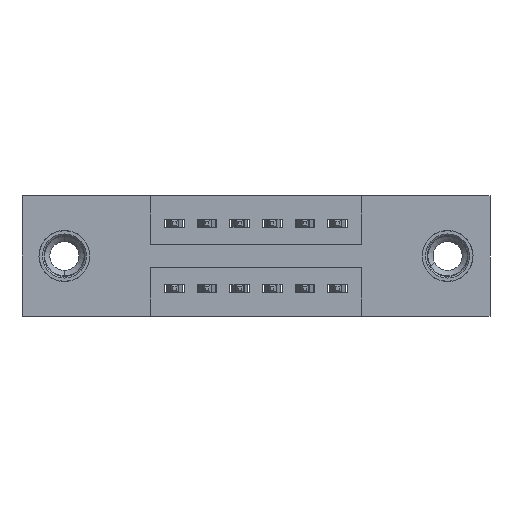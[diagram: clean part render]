
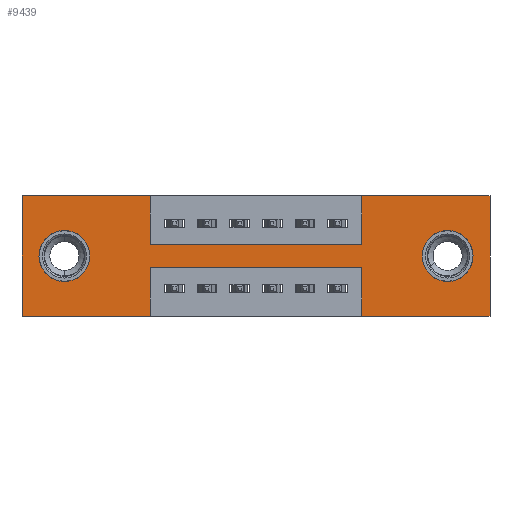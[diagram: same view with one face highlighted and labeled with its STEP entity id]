
A CAD part, front view. The second image highlights one B-rep face of the part: STEP entity #9439.
In plain terms, the highlighted planar face has unit normal (0, -1, 0).
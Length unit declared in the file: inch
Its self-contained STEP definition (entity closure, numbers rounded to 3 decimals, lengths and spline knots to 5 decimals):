
#86 = VERTEX_POINT ( 'NONE', #9624 ) ;
#166 = CARTESIAN_POINT ( 'NONE',  ( 1.305, 0., -0.107 ) ) ;
#255 = LINE ( 'NONE', #271, #2035 ) ;
#271 = CARTESIAN_POINT ( 'NONE',  ( 0., 0., -0.37 ) ) ;
#305 = DIRECTION ( 'NONE',  ( 0., 1., 0. ) ) ;
#328 = EDGE_CURVE ( 'NONE', #8763, #6198, #1957, .T. ) ;
#438 = CARTESIAN_POINT ( 'NONE',  ( 0., 0., -0.37 ) ) ;
#487 = EDGE_CURVE ( 'NONE', #9797, #8559, #4490, .T. ) ;
#551 = DIRECTION ( 'NONE',  ( 0., 0., 1. ) ) ;
#557 = EDGE_CURVE ( 'NONE', #3294, #9797, #3960, .T. ) ;
#584 = LINE ( 'NONE', #10082, #9208 ) ;
#622 = VERTEX_POINT ( 'NONE', #3909 ) ;
#624 = DIRECTION ( 'NONE',  ( 0., 0., -1. ) ) ;
#631 = CARTESIAN_POINT ( 'NONE',  ( 1.435, 0., 0. ) ) ;
#964 = AXIS2_PLACEMENT_3D ( 'NONE', #2836, #305, #3231 ) ;
#1215 = DIRECTION ( 'NONE',  ( 0., 1., 0. ) ) ;
#1253 = CARTESIAN_POINT ( 'NONE',  ( 1.0425, 0., -0.37 ) ) ;
#1307 = CARTESIAN_POINT ( 'NONE',  ( 0., 0., 0. ) ) ;
#1311 = VERTEX_POINT ( 'NONE', #1877 ) ;
#1319 = EDGE_LOOP ( 'NONE', ( #7394, #8394 ) ) ;
#1360 = VECTOR ( 'NONE', #5680, 39.37008 ) ;
#1423 = EDGE_CURVE ( 'NONE', #2237, #2375, #4762, .T. ) ;
#1459 = CARTESIAN_POINT ( 'NONE',  ( 0., 0., -0.37 ) ) ;
#1577 = LINE ( 'NONE', #1459, #7992 ) ;
#1595 = CIRCLE ( 'NONE', #5994, 0.078 ) ;
#1633 = EDGE_CURVE ( 'NONE', #3904, #86, #584, .T. ) ;
#1877 = CARTESIAN_POINT ( 'NONE',  ( 1.435, 0., -0.37 ) ) ;
#1957 = CIRCLE ( 'NONE', #10383, 0.078 ) ;
#1965 = VECTOR ( 'NONE', #6711, 39.37008 ) ;
#2035 = VECTOR ( 'NONE', #6252, 39.37008 ) ;
#2062 = LINE ( 'NONE', #9453, #10078 ) ;
#2091 = CARTESIAN_POINT ( 'NONE',  ( 0., 0., 0. ) ) ;
#2122 = VERTEX_POINT ( 'NONE', #5697 ) ;
#2140 = ORIENTED_EDGE ( 'NONE', *, *, #9640, .F. ) ;
#2146 = VERTEX_POINT ( 'NONE', #166 ) ;
#2157 = LINE ( 'NONE', #2091, #8541 ) ;
#2207 = EDGE_CURVE ( 'NONE', #86, #2122, #2062, .T. ) ;
#2211 = FACE_BOUND ( 'NONE', #1319, .T. ) ;
#2237 = VERTEX_POINT ( 'NONE', #9312 ) ;
#2335 = CARTESIAN_POINT ( 'NONE',  ( 0.3925, 0., 0. ) ) ;
#2375 = VERTEX_POINT ( 'NONE', #4013 ) ;
#2468 = VECTOR ( 'NONE', #4697, 39.37008 ) ;
#2488 = VERTEX_POINT ( 'NONE', #10717 ) ;
#2558 = DIRECTION ( 'NONE',  ( 0., 1., 0. ) ) ;
#2757 = CARTESIAN_POINT ( 'NONE',  ( 0.13, 0., -0.185 ) ) ;
#2765 = EDGE_CURVE ( 'NONE', #2146, #7243, #5010, .T. ) ;
#2836 = CARTESIAN_POINT ( 'NONE',  ( 1.305, 0., -0.185 ) ) ;
#2976 = DIRECTION ( 'NONE',  ( 0., 0., 1. ) ) ;
#3026 = CARTESIAN_POINT ( 'NONE',  ( 1.305, 0., -0.263 ) ) ;
#3231 = DIRECTION ( 'NONE',  ( 0., 0., -1. ) ) ;
#3263 = CARTESIAN_POINT ( 'NONE',  ( 0.13, 0., -0.107 ) ) ;
#3294 = VERTEX_POINT ( 'NONE', #8430 ) ;
#3357 = VECTOR ( 'NONE', #5086, 39.37008 ) ;
#3497 = LINE ( 'NONE', #1253, #9552 ) ;
#3625 = DIRECTION ( 'NONE',  ( 0., 0., 1. ) ) ;
#3855 = EDGE_CURVE ( 'NONE', #8559, #1311, #10166, .T. ) ;
#3904 = VERTEX_POINT ( 'NONE', #5490 ) ;
#3909 = CARTESIAN_POINT ( 'NONE',  ( 0., 0., 0. ) ) ;
#3960 = LINE ( 'NONE', #7753, #1965 ) ;
#4013 = CARTESIAN_POINT ( 'NONE',  ( 0.3925, 0., -0.15 ) ) ;
#4252 = ORIENTED_EDGE ( 'NONE', *, *, #4639, .F. ) ;
#4260 = EDGE_CURVE ( 'NONE', #2375, #3294, #8279, .T. ) ;
#4428 = DIRECTION ( 'NONE',  ( 0., -1., 0. ) ) ;
#4490 = LINE ( 'NONE', #7725, #8617 ) ;
#4499 = EDGE_LOOP ( 'NONE', ( #5506, #5507 ) ) ;
#4639 = EDGE_CURVE ( 'NONE', #2122, #8376, #255, .T. ) ;
#4697 = DIRECTION ( 'NONE',  ( 0., 0., -1. ) ) ;
#4762 = LINE ( 'NONE', #2335, #2468 ) ;
#5010 = CIRCLE ( 'NONE', #964, 0.078 ) ;
#5086 = DIRECTION ( 'NONE',  ( 0., 0., -1. ) ) ;
#5281 = CARTESIAN_POINT ( 'NONE',  ( 0., 0., -0.37 ) ) ;
#5383 = ORIENTED_EDGE ( 'NONE', *, *, #5393, .F. ) ;
#5393 = EDGE_CURVE ( 'NONE', #622, #2237, #2157, .T. ) ;
#5490 = CARTESIAN_POINT ( 'NONE',  ( 1.0425, 0., -0.22 ) ) ;
#5506 = ORIENTED_EDGE ( 'NONE', *, *, #2765, .T. ) ;
#5507 = ORIENTED_EDGE ( 'NONE', *, *, #8921, .T. ) ;
#5510 = DIRECTION ( 'NONE',  ( 1., 0., 0. ) ) ;
#5520 = ORIENTED_EDGE ( 'NONE', *, *, #2207, .F. ) ;
#5680 = DIRECTION ( 'NONE',  ( 1., 0., 0. ) ) ;
#5697 = CARTESIAN_POINT ( 'NONE',  ( 0.3925, 0., -0.37 ) ) ;
#5874 = EDGE_LOOP ( 'NONE', ( #5520, #6567, #6012, #9488, #7519, #8018, #7683, #7933, #6992, #5383, #2140, #4252 ) ) ;
#5994 = AXIS2_PLACEMENT_3D ( 'NONE', #2757, #8583, #3625 ) ;
#6012 = ORIENTED_EDGE ( 'NONE', *, *, #10746, .F. ) ;
#6198 = VERTEX_POINT ( 'NONE', #3263 ) ;
#6252 = DIRECTION ( 'NONE',  ( -1., 0., 0. ) ) ;
#6277 = CARTESIAN_POINT ( 'NONE',  ( 1.305, 0., -0.185 ) ) ;
#6309 = DIRECTION ( 'NONE',  ( 0., 0., 1. ) ) ;
#6567 = ORIENTED_EDGE ( 'NONE', *, *, #1633, .F. ) ;
#6635 = CARTESIAN_POINT ( 'NONE',  ( 1.435, 0., 0. ) ) ;
#6711 = DIRECTION ( 'NONE',  ( 0., 0., 1. ) ) ;
#6794 = LINE ( 'NONE', #1307, #10561 ) ;
#6926 = CARTESIAN_POINT ( 'NONE',  ( 0.13, 0., -0.185 ) ) ;
#6992 = ORIENTED_EDGE ( 'NONE', *, *, #1423, .F. ) ;
#6998 = EDGE_CURVE ( 'NONE', #6198, #8763, #1595, .T. ) ;
#7068 = DIRECTION ( 'NONE',  ( 0., 0., -1. ) ) ;
#7243 = VERTEX_POINT ( 'NONE', #3026 ) ;
#7394 = ORIENTED_EDGE ( 'NONE', *, *, #6998, .T. ) ;
#7519 = ORIENTED_EDGE ( 'NONE', *, *, #3855, .F. ) ;
#7683 = ORIENTED_EDGE ( 'NONE', *, *, #557, .F. ) ;
#7697 = AXIS2_PLACEMENT_3D ( 'NONE', #5281, #4428, #10136 ) ;
#7725 = CARTESIAN_POINT ( 'NONE',  ( 0., 0., 0. ) ) ;
#7753 = CARTESIAN_POINT ( 'NONE',  ( 1.0425, 0., 0. ) ) ;
#7933 = ORIENTED_EDGE ( 'NONE', *, *, #4260, .F. ) ;
#7956 = EDGE_CURVE ( 'NONE', #1311, #2488, #1577, .T. ) ;
#7992 = VECTOR ( 'NONE', #8952, 39.37008 ) ;
#8018 = ORIENTED_EDGE ( 'NONE', *, *, #487, .F. ) ;
#8137 = DIRECTION ( 'NONE',  ( -1., 0., 0. ) ) ;
#8279 = LINE ( 'NONE', #10456, #1360 ) ;
#8376 = VERTEX_POINT ( 'NONE', #438 ) ;
#8394 = ORIENTED_EDGE ( 'NONE', *, *, #328, .T. ) ;
#8430 = CARTESIAN_POINT ( 'NONE',  ( 1.0425, 0., -0.15 ) ) ;
#8541 = VECTOR ( 'NONE', #5510, 39.37008 ) ;
#8559 = VERTEX_POINT ( 'NONE', #631 ) ;
#8583 = DIRECTION ( 'NONE',  ( 0., 1., 0. ) ) ;
#8589 = FACE_BOUND ( 'NONE', #4499, .T. ) ;
#8617 = VECTOR ( 'NONE', #9157, 39.37008 ) ;
#8763 = VERTEX_POINT ( 'NONE', #9207 ) ;
#8849 = FACE_OUTER_BOUND ( 'NONE', #5874, .T. ) ;
#8921 = EDGE_CURVE ( 'NONE', #7243, #2146, #9591, .T. ) ;
#8952 = DIRECTION ( 'NONE',  ( -1., 0., 0. ) ) ;
#8987 = CARTESIAN_POINT ( 'NONE',  ( 1.0425, 0., 0. ) ) ;
#9157 = DIRECTION ( 'NONE',  ( 1., 0., 0. ) ) ;
#9207 = CARTESIAN_POINT ( 'NONE',  ( 0.13, 0., -0.263 ) ) ;
#9208 = VECTOR ( 'NONE', #8137, 39.37008 ) ;
#9312 = CARTESIAN_POINT ( 'NONE',  ( 0.3925, 0., 0. ) ) ;
#9333 = PLANE ( 'NONE',  #7697 ) ;
#9439 = ADVANCED_FACE ( 'NONE', ( #8589, #2211, #8849 ), #9333, .T. ) ;
#9453 = CARTESIAN_POINT ( 'NONE',  ( 0.3925, 0., -0.37 ) ) ;
#9488 = ORIENTED_EDGE ( 'NONE', *, *, #7956, .F. ) ;
#9552 = VECTOR ( 'NONE', #6309, 39.37008 ) ;
#9591 = CIRCLE ( 'NONE', #10254, 0.078 ) ;
#9624 = CARTESIAN_POINT ( 'NONE',  ( 0.3925, 0., -0.22 ) ) ;
#9640 = EDGE_CURVE ( 'NONE', #8376, #622, #6794, .T. ) ;
#9797 = VERTEX_POINT ( 'NONE', #8987 ) ;
#10078 = VECTOR ( 'NONE', #624, 39.37008 ) ;
#10082 = CARTESIAN_POINT ( 'NONE',  ( 0.3925, 0., -0.22 ) ) ;
#10136 = DIRECTION ( 'NONE',  ( 0., 0., -1. ) ) ;
#10166 = LINE ( 'NONE', #6635, #3357 ) ;
#10254 = AXIS2_PLACEMENT_3D ( 'NONE', #6277, #1215, #7068 ) ;
#10383 = AXIS2_PLACEMENT_3D ( 'NONE', #6926, #2558, #551 ) ;
#10456 = CARTESIAN_POINT ( 'NONE',  ( 0.3925, 0., -0.15 ) ) ;
#10561 = VECTOR ( 'NONE', #2976, 39.37008 ) ;
#10717 = CARTESIAN_POINT ( 'NONE',  ( 1.0425, 0., -0.37 ) ) ;
#10746 = EDGE_CURVE ( 'NONE', #2488, #3904, #3497, .T. ) ;
